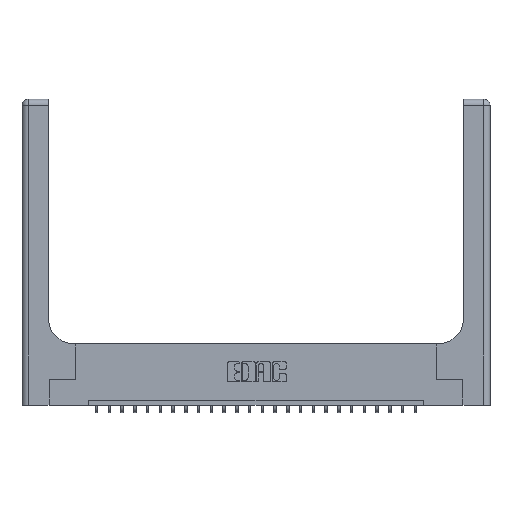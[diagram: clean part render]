
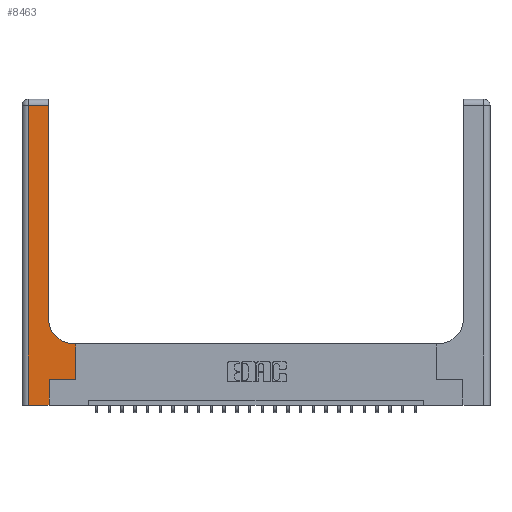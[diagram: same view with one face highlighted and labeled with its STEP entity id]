
A CAD part, top view. The second image highlights one B-rep face of the part: STEP entity #8463.
In plain terms, the highlighted planar face has unit normal (0, 0, 1).
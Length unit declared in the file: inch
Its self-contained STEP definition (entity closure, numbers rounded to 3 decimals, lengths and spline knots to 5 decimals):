
#555 = CARTESIAN_POINT ( 'NONE',  ( 0.26, 0.85, 0.37 ) ) ;
#659 = EDGE_CURVE ( 'NONE', #9596, #16086, #889, .T. ) ;
#702 = ORIENTED_EDGE ( 'NONE', *, *, #22317, .T. ) ;
#793 = CARTESIAN_POINT ( 'NONE',  ( 0.51, 0.6, 0.37 ) ) ;
#889 = LINE ( 'NONE', #19298, #15471 ) ;
#981 = CIRCLE ( 'NONE', #15164, 0.25 ) ;
#1054 = DIRECTION ( 'NONE',  ( 1., 0., 0. ) ) ;
#1219 = DIRECTION ( 'NONE',  ( 1., 0., 0. ) ) ;
#1661 = ORIENTED_EDGE ( 'NONE', *, *, #22357, .T. ) ;
#1765 = CARTESIAN_POINT ( 'NONE',  ( 0.26, 0.6, 0.37 ) ) ;
#1873 = VERTEX_POINT ( 'NONE', #12063 ) ;
#2429 = DIRECTION ( 'NONE',  ( 0., 1., 0. ) ) ;
#2528 = EDGE_CURVE ( 'NONE', #9446, #1873, #20842, .T. ) ;
#2542 = VERTEX_POINT ( 'NONE', #15829 ) ;
#2692 = CARTESIAN_POINT ( 'NONE',  ( 0.51, 0.85, 0.37 ) ) ;
#2695 = CARTESIAN_POINT ( 'NONE',  ( 0., 3., 0.37 ) ) ;
#2727 = LINE ( 'NONE', #18774, #11855 ) ;
#3565 = DIRECTION ( 'NONE',  ( 0., 1., 0. ) ) ;
#3752 = ORIENTED_EDGE ( 'NONE', *, *, #6551, .T. ) ;
#3932 = VECTOR ( 'NONE', #7824, 39.37008 ) ;
#4270 = DIRECTION ( 'NONE',  ( 0., 1., 0. ) ) ;
#4549 = DIRECTION ( 'NONE',  ( 1., 0., 0. ) ) ;
#4580 = CARTESIAN_POINT ( 'NONE',  ( 0.26, 2.94, 0.37 ) ) ;
#5258 = LINE ( 'NONE', #7283, #10100 ) ;
#5464 = EDGE_CURVE ( 'NONE', #16086, #15438, #22973, .T. ) ;
#6398 = DIRECTION ( 'NONE',  ( -1., 0., 0. ) ) ;
#6416 = VECTOR ( 'NONE', #1219, 39.37008 ) ;
#6551 = EDGE_CURVE ( 'NONE', #2542, #9446, #15897, .T. ) ;
#7023 = ORIENTED_EDGE ( 'NONE', *, *, #659, .T. ) ;
#7283 = CARTESIAN_POINT ( 'NONE',  ( 0.265, 0., 0.37 ) ) ;
#7630 = EDGE_CURVE ( 'NONE', #18689, #2542, #17821, .T. ) ;
#7824 = DIRECTION ( 'NONE',  ( -1., 0., 0. ) ) ;
#7900 = CARTESIAN_POINT ( 'NONE',  ( 0.528, 0.25, 0.37 ) ) ;
#8463 = ADVANCED_FACE ( 'NONE', ( #17623 ), #15427, .F. ) ;
#8584 = CARTESIAN_POINT ( 'NONE',  ( 0., 0., 0.37 ) ) ;
#8614 = VECTOR ( 'NONE', #2429, 39.37008 ) ;
#8644 = CARTESIAN_POINT ( 'NONE',  ( 0.06, 3., 0.37 ) ) ;
#9446 = VERTEX_POINT ( 'NONE', #10893 ) ;
#9543 = VECTOR ( 'NONE', #14523, 39.37008 ) ;
#9596 = VERTEX_POINT ( 'NONE', #16661 ) ;
#9598 = EDGE_LOOP ( 'NONE', ( #14403, #11985, #3752, #20456, #702, #7023, #22353, #1661, #21312 ) ) ;
#10100 = VECTOR ( 'NONE', #3565, 39.37008 ) ;
#10513 = CARTESIAN_POINT ( 'NONE',  ( 0.528, 0.6, 0.37 ) ) ;
#10893 = CARTESIAN_POINT ( 'NONE',  ( 0.06, 0., 0.37 ) ) ;
#11855 = VECTOR ( 'NONE', #4270, 39.37008 ) ;
#11985 = ORIENTED_EDGE ( 'NONE', *, *, #7630, .T. ) ;
#12063 = CARTESIAN_POINT ( 'NONE',  ( 0.265, 0., 0.37 ) ) ;
#13225 = VERTEX_POINT ( 'NONE', #793 ) ;
#13996 = DIRECTION ( 'NONE',  ( 0., -1., 0. ) ) ;
#14403 = ORIENTED_EDGE ( 'NONE', *, *, #20845, .T. ) ;
#14523 = DIRECTION ( 'NONE',  ( -1., 0., 0. ) ) ;
#15057 = CARTESIAN_POINT ( 'NONE',  ( 0., 2.94, 0.37 ) ) ;
#15164 = AXIS2_PLACEMENT_3D ( 'NONE', #2692, #15423, #4549 ) ;
#15206 = EDGE_CURVE ( 'NONE', #13225, #19586, #981, .T. ) ;
#15423 = DIRECTION ( 'NONE',  ( 0., 0., -1. ) ) ;
#15427 = PLANE ( 'NONE',  #20075 ) ;
#15438 = VERTEX_POINT ( 'NONE', #10513 ) ;
#15471 = VECTOR ( 'NONE', #1054, 39.37008 ) ;
#15829 = CARTESIAN_POINT ( 'NONE',  ( 0.06, 2.94, 0.37 ) ) ;
#15897 = LINE ( 'NONE', #8644, #20691 ) ;
#16086 = VERTEX_POINT ( 'NONE', #7900 ) ;
#16661 = CARTESIAN_POINT ( 'NONE',  ( 0.265, 0.25, 0.37 ) ) ;
#17229 = DIRECTION ( 'NONE',  ( 0., 0., -1. ) ) ;
#17623 = FACE_OUTER_BOUND ( 'NONE', #9598, .T. ) ;
#17821 = LINE ( 'NONE', #15057, #3932 ) ;
#18689 = VERTEX_POINT ( 'NONE', #4580 ) ;
#18774 = CARTESIAN_POINT ( 'NONE',  ( 0.26, 3., 0.37 ) ) ;
#19298 = CARTESIAN_POINT ( 'NONE',  ( 0.265, 0.25, 0.37 ) ) ;
#19586 = VERTEX_POINT ( 'NONE', #555 ) ;
#20075 = AXIS2_PLACEMENT_3D ( 'NONE', #2695, #17229, #6398 ) ;
#20261 = LINE ( 'NONE', #1765, #9543 ) ;
#20456 = ORIENTED_EDGE ( 'NONE', *, *, #2528, .T. ) ;
#20691 = VECTOR ( 'NONE', #13996, 39.37008 ) ;
#20842 = LINE ( 'NONE', #8584, #6416 ) ;
#20845 = EDGE_CURVE ( 'NONE', #19586, #18689, #2727, .T. ) ;
#21312 = ORIENTED_EDGE ( 'NONE', *, *, #15206, .T. ) ;
#22317 = EDGE_CURVE ( 'NONE', #1873, #9596, #5258, .T. ) ;
#22326 = CARTESIAN_POINT ( 'NONE',  ( 0.528, 0.25, 0.37 ) ) ;
#22353 = ORIENTED_EDGE ( 'NONE', *, *, #5464, .T. ) ;
#22357 = EDGE_CURVE ( 'NONE', #15438, #13225, #20261, .T. ) ;
#22973 = LINE ( 'NONE', #22326, #8614 ) ;
